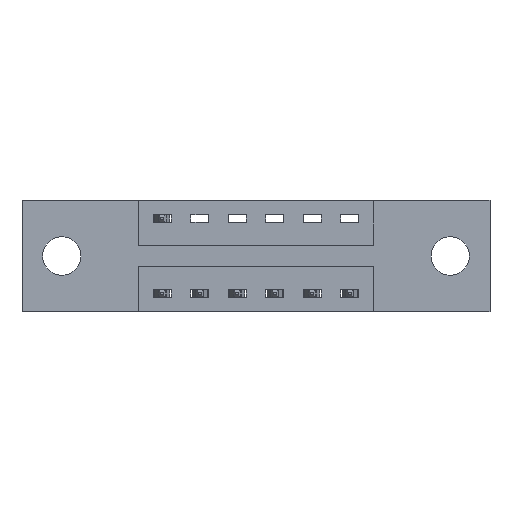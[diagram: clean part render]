
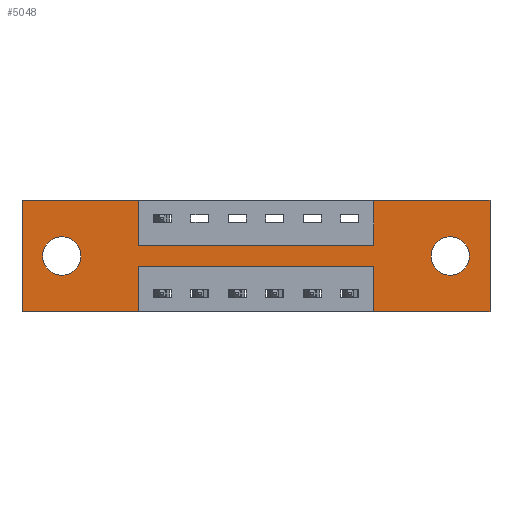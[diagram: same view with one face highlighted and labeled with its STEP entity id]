
A CAD part, front view. The second image highlights one B-rep face of the part: STEP entity #5048.
In plain terms, the highlighted planar face has unit normal (0, -1, 0).
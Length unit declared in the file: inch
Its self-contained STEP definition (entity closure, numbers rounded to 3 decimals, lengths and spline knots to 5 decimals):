
#304 = EDGE_CURVE ( 'NONE', #7312, #4621, #7618, .T. ) ;
#319 = VERTEX_POINT ( 'NONE', #6707 ) ;
#370 = EDGE_CURVE ( 'NONE', #3397, #1192, #6966, .T. ) ;
#506 = CARTESIAN_POINT ( 'NONE',  ( 0.3875, 0., -0.15 ) ) ;
#623 = EDGE_CURVE ( 'NONE', #1240, #6071, #5147, .T. ) ;
#661 = AXIS2_PLACEMENT_3D ( 'NONE', #2941, #7525, #3616 ) ;
#896 = DIRECTION ( 'NONE',  ( 0., 1., 0. ) ) ;
#1067 = DIRECTION ( 'NONE',  ( 0., 1., 0. ) ) ;
#1192 = VERTEX_POINT ( 'NONE', #6105 ) ;
#1240 = VERTEX_POINT ( 'NONE', #5971 ) ;
#1335 = VERTEX_POINT ( 'NONE', #3628 ) ;
#1411 = LINE ( 'NONE', #1790, #6240 ) ;
#1442 = FACE_BOUND ( 'NONE', #7703, .T. ) ;
#1601 = CARTESIAN_POINT ( 'NONE',  ( 1.1725, 0., -0.37 ) ) ;
#1640 = VECTOR ( 'NONE', #6891, 39.37008 ) ;
#1710 = LINE ( 'NONE', #7891, #6752 ) ;
#1740 = EDGE_LOOP ( 'NONE', ( #6875, #5475, #7846, #7129, #6910, #7328, #8108, #7362, #7480, #6828, #7649, #8375 ) ) ;
#1759 = EDGE_CURVE ( 'NONE', #3496, #1240, #1411, .T. ) ;
#1790 = CARTESIAN_POINT ( 'NONE',  ( 1.56, 0., 0. ) ) ;
#1820 = DIRECTION ( 'NONE',  ( 0., 1., 0. ) ) ;
#1889 = EDGE_CURVE ( 'NONE', #6629, #5107, #1710, .T. ) ;
#1904 = DIRECTION ( 'NONE',  ( 0., 0., -1. ) ) ;
#2191 = EDGE_CURVE ( 'NONE', #1192, #3496, #6428, .T. ) ;
#2305 = AXIS2_PLACEMENT_3D ( 'NONE', #3556, #1067, #6044 ) ;
#2320 = DIRECTION ( 'NONE',  ( -1., 0., 0. ) ) ;
#2325 = VERTEX_POINT ( 'NONE', #2540 ) ;
#2346 = DIRECTION ( 'NONE',  ( -1., 0., 0. ) ) ;
#2425 = CARTESIAN_POINT ( 'NONE',  ( 0., 0., 0. ) ) ;
#2540 = CARTESIAN_POINT ( 'NONE',  ( 0., 0., 0. ) ) ;
#2679 = CARTESIAN_POINT ( 'NONE',  ( 1.1725, 0., 0. ) ) ;
#2716 = EDGE_CURVE ( 'NONE', #3980, #2325, #8301, .T. ) ;
#2941 = CARTESIAN_POINT ( 'NONE',  ( 0.1325, 0., -0.185 ) ) ;
#2976 = CIRCLE ( 'NONE', #4140, 0.064 ) ;
#2996 = VECTOR ( 'NONE', #4541, 39.37008 ) ;
#3022 = FACE_OUTER_BOUND ( 'NONE', #1740, .T. ) ;
#3068 = VECTOR ( 'NONE', #3710, 39.37008 ) ;
#3143 = DIRECTION ( 'NONE',  ( 0., 0., -1. ) ) ;
#3254 = DIRECTION ( 'NONE',  ( 0., 0., 1. ) ) ;
#3397 = VERTEX_POINT ( 'NONE', #5676 ) ;
#3431 = LINE ( 'NONE', #5775, #2996 ) ;
#3496 = VERTEX_POINT ( 'NONE', #5793 ) ;
#3525 = LINE ( 'NONE', #6907, #6766 ) ;
#3556 = CARTESIAN_POINT ( 'NONE',  ( 0.1325, 0., -0.185 ) ) ;
#3558 = VECTOR ( 'NONE', #5194, 39.37008 ) ;
#3616 = DIRECTION ( 'NONE',  ( 0., 0., 1. ) ) ;
#3628 = CARTESIAN_POINT ( 'NONE',  ( 1.4275, 0., -0.121 ) ) ;
#3710 = DIRECTION ( 'NONE',  ( 0., 0., 1. ) ) ;
#3723 = CARTESIAN_POINT ( 'NONE',  ( 1.4275, 0., -0.249 ) ) ;
#3837 = CARTESIAN_POINT ( 'NONE',  ( 0., 0., 0. ) ) ;
#3971 = CARTESIAN_POINT ( 'NONE',  ( 0.3875, 0., -0.22 ) ) ;
#3980 = VERTEX_POINT ( 'NONE', #6258 ) ;
#4140 = AXIS2_PLACEMENT_3D ( 'NONE', #5766, #1820, #6403 ) ;
#4214 = EDGE_CURVE ( 'NONE', #319, #3397, #5285, .T. ) ;
#4541 = DIRECTION ( 'NONE',  ( 0., 0., -1. ) ) ;
#4621 = VERTEX_POINT ( 'NONE', #4827 ) ;
#4645 = VECTOR ( 'NONE', #6424, 39.37008 ) ;
#4827 = CARTESIAN_POINT ( 'NONE',  ( 0.1325, 0., -0.121 ) ) ;
#4855 = CARTESIAN_POINT ( 'NONE',  ( 0., 0., -0.37 ) ) ;
#4904 = CARTESIAN_POINT ( 'NONE',  ( 1.4275, 0., -0.185 ) ) ;
#4945 = VECTOR ( 'NONE', #5440, 39.37008 ) ;
#4953 = DIRECTION ( 'NONE',  ( 0., 0., 1. ) ) ;
#5048 = ADVANCED_FACE ( 'NONE', ( #1442, #6473, #3022 ), #5207, .T. ) ;
#5107 = VERTEX_POINT ( 'NONE', #3971 ) ;
#5147 = LINE ( 'NONE', #4855, #4945 ) ;
#5194 = DIRECTION ( 'NONE',  ( 1., 0., 0. ) ) ;
#5207 = PLANE ( 'NONE',  #5952 ) ;
#5285 = LINE ( 'NONE', #506, #3558 ) ;
#5440 = DIRECTION ( 'NONE',  ( -1., 0., 0. ) ) ;
#5475 = ORIENTED_EDGE ( 'NONE', *, *, #1889, .F. ) ;
#5479 = EDGE_CURVE ( 'NONE', #8395, #319, #6878, .T. ) ;
#5538 = DIRECTION ( 'NONE',  ( 0., 0., -1. ) ) ;
#5676 = CARTESIAN_POINT ( 'NONE',  ( 1.1725, 0., -0.15 ) ) ;
#5766 = CARTESIAN_POINT ( 'NONE',  ( 1.4275, 0., -0.185 ) ) ;
#5775 = CARTESIAN_POINT ( 'NONE',  ( 0.3875, 0., -0.37 ) ) ;
#5793 = CARTESIAN_POINT ( 'NONE',  ( 1.56, 0., 0. ) ) ;
#5859 = DIRECTION ( 'NONE',  ( 0., -1., 0. ) ) ;
#5952 = AXIS2_PLACEMENT_3D ( 'NONE', #7836, #5859, #1904 ) ;
#5971 = CARTESIAN_POINT ( 'NONE',  ( 1.56, 0., -0.37 ) ) ;
#6044 = DIRECTION ( 'NONE',  ( 0., 0., 1. ) ) ;
#6071 = VERTEX_POINT ( 'NONE', #1601 ) ;
#6105 = CARTESIAN_POINT ( 'NONE',  ( 1.1725, 0., 0. ) ) ;
#6131 = EDGE_CURVE ( 'NONE', #7657, #3980, #3525, .T. ) ;
#6236 = CARTESIAN_POINT ( 'NONE',  ( 0.3875, 0., 0. ) ) ;
#6240 = VECTOR ( 'NONE', #3143, 39.37008 ) ;
#6258 = CARTESIAN_POINT ( 'NONE',  ( 0., 0., -0.37 ) ) ;
#6291 = EDGE_CURVE ( 'NONE', #5107, #7657, #3431, .T. ) ;
#6323 = LINE ( 'NONE', #3837, #4645 ) ;
#6334 = EDGE_CURVE ( 'NONE', #6071, #6629, #7833, .T. ) ;
#6343 = DIRECTION ( 'NONE',  ( 1., 0., 0. ) ) ;
#6403 = DIRECTION ( 'NONE',  ( 0., 0., -1. ) ) ;
#6424 = DIRECTION ( 'NONE',  ( 1., 0., 0. ) ) ;
#6427 = CIRCLE ( 'NONE', #661, 0.064 ) ;
#6428 = LINE ( 'NONE', #2425, #8019 ) ;
#6473 = FACE_BOUND ( 'NONE', #7017, .T. ) ;
#6492 = ORIENTED_EDGE ( 'NONE', *, *, #7636, .T. ) ;
#6614 = CARTESIAN_POINT ( 'NONE',  ( 0.3875, 0., 0. ) ) ;
#6623 = EDGE_CURVE ( 'NONE', #7313, #1335, #7058, .T. ) ;
#6629 = VERTEX_POINT ( 'NONE', #7496 ) ;
#6707 = CARTESIAN_POINT ( 'NONE',  ( 0.3875, 0., -0.15 ) ) ;
#6718 = ORIENTED_EDGE ( 'NONE', *, *, #6623, .T. ) ;
#6752 = VECTOR ( 'NONE', #2320, 39.37008 ) ;
#6766 = VECTOR ( 'NONE', #2346, 39.37008 ) ;
#6828 = ORIENTED_EDGE ( 'NONE', *, *, #7435, .F. ) ;
#6875 = ORIENTED_EDGE ( 'NONE', *, *, #6291, .F. ) ;
#6878 = LINE ( 'NONE', #6236, #1640 ) ;
#6891 = DIRECTION ( 'NONE',  ( 0., 0., -1. ) ) ;
#6907 = CARTESIAN_POINT ( 'NONE',  ( 0., 0., -0.37 ) ) ;
#6910 = ORIENTED_EDGE ( 'NONE', *, *, #1759, .F. ) ;
#6934 = CARTESIAN_POINT ( 'NONE',  ( 0., 0., 0. ) ) ;
#6966 = LINE ( 'NONE', #2679, #8535 ) ;
#7017 = EDGE_LOOP ( 'NONE', ( #7658, #7623 ) ) ;
#7058 = CIRCLE ( 'NONE', #7807, 0.064 ) ;
#7129 = ORIENTED_EDGE ( 'NONE', *, *, #623, .F. ) ;
#7183 = EDGE_CURVE ( 'NONE', #4621, #7312, #6427, .T. ) ;
#7312 = VERTEX_POINT ( 'NONE', #7641 ) ;
#7313 = VERTEX_POINT ( 'NONE', #3723 ) ;
#7328 = ORIENTED_EDGE ( 'NONE', *, *, #2191, .F. ) ;
#7362 = ORIENTED_EDGE ( 'NONE', *, *, #4214, .F. ) ;
#7435 = EDGE_CURVE ( 'NONE', #2325, #8395, #6323, .T. ) ;
#7480 = ORIENTED_EDGE ( 'NONE', *, *, #5479, .F. ) ;
#7496 = CARTESIAN_POINT ( 'NONE',  ( 1.1725, 0., -0.22 ) ) ;
#7525 = DIRECTION ( 'NONE',  ( 0., 1., 0. ) ) ;
#7611 = VECTOR ( 'NONE', #3254, 39.37008 ) ;
#7618 = CIRCLE ( 'NONE', #2305, 0.064 ) ;
#7623 = ORIENTED_EDGE ( 'NONE', *, *, #304, .T. ) ;
#7636 = EDGE_CURVE ( 'NONE', #1335, #7313, #2976, .T. ) ;
#7641 = CARTESIAN_POINT ( 'NONE',  ( 0.1325, 0., -0.249 ) ) ;
#7649 = ORIENTED_EDGE ( 'NONE', *, *, #2716, .F. ) ;
#7657 = VERTEX_POINT ( 'NONE', #7774 ) ;
#7658 = ORIENTED_EDGE ( 'NONE', *, *, #7183, .T. ) ;
#7703 = EDGE_LOOP ( 'NONE', ( #6492, #6718 ) ) ;
#7774 = CARTESIAN_POINT ( 'NONE',  ( 0.3875, 0., -0.37 ) ) ;
#7807 = AXIS2_PLACEMENT_3D ( 'NONE', #4904, #896, #5538 ) ;
#7833 = LINE ( 'NONE', #8455, #7611 ) ;
#7836 = CARTESIAN_POINT ( 'NONE',  ( 0., 0., -0.37 ) ) ;
#7846 = ORIENTED_EDGE ( 'NONE', *, *, #6334, .F. ) ;
#7891 = CARTESIAN_POINT ( 'NONE',  ( 0.3875, 0., -0.22 ) ) ;
#8019 = VECTOR ( 'NONE', #6343, 39.37008 ) ;
#8108 = ORIENTED_EDGE ( 'NONE', *, *, #370, .F. ) ;
#8301 = LINE ( 'NONE', #6934, #3068 ) ;
#8375 = ORIENTED_EDGE ( 'NONE', *, *, #6131, .F. ) ;
#8395 = VERTEX_POINT ( 'NONE', #6614 ) ;
#8455 = CARTESIAN_POINT ( 'NONE',  ( 1.1725, 0., -0.37 ) ) ;
#8535 = VECTOR ( 'NONE', #4953, 39.37008 ) ;
